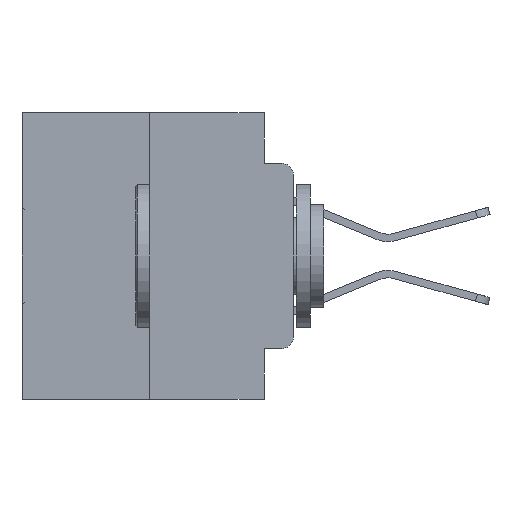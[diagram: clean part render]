
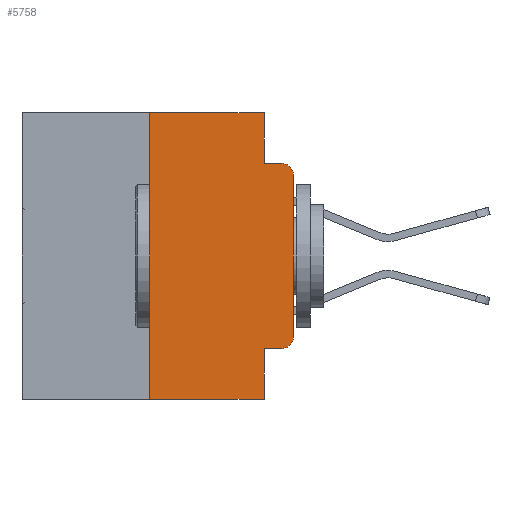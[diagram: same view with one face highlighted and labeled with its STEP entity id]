
A CAD part, left-side view. The second image highlights one B-rep face of the part: STEP entity #5758.
In plain terms, the highlighted planar face has unit normal (-1, 0, 0).
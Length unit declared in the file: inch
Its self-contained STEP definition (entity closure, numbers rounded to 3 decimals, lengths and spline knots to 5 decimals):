
#110 = ORIENTED_EDGE ( 'NONE', *, *, #951, .T. ) ;
#783 = VERTEX_POINT ( 'NONE', #11656 ) ;
#951 = EDGE_CURVE ( 'NONE', #11576, #783, #6256, .T. ) ;
#1330 = CARTESIAN_POINT ( 'NONE',  ( 0., 0., -0.1085 ) ) ;
#1408 = CARTESIAN_POINT ( 'NONE',  ( 0., 0.051, -0.4115 ) ) ;
#1861 = DIRECTION ( 'NONE',  ( 0., -1., 0. ) ) ;
#2162 = LINE ( 'NONE', #21679, #14108 ) ;
#2329 = ORIENTED_EDGE ( 'NONE', *, *, #25885, .T. ) ;
#2537 = ORIENTED_EDGE ( 'NONE', *, *, #22961, .T. ) ;
#3094 = VECTOR ( 'NONE', #11346, 39.37008 ) ;
#3919 = CARTESIAN_POINT ( 'NONE',  ( 0., 0.051, 0. ) ) ;
#4466 = ORIENTED_EDGE ( 'NONE', *, *, #26019, .F. ) ;
#4568 = VERTEX_POINT ( 'NONE', #19889 ) ;
#4590 = CARTESIAN_POINT ( 'NONE',  ( 0., 0.051, -0.0885 ) ) ;
#4598 = VECTOR ( 'NONE', #23918, 39.37008 ) ;
#4749 = LINE ( 'NONE', #4590, #29513 ) ;
#4947 = VECTOR ( 'NONE', #23850, 39.37008 ) ;
#5652 = CARTESIAN_POINT ( 'NONE',  ( 0., 0.473, 0. ) ) ;
#5730 = VERTEX_POINT ( 'NONE', #3919 ) ;
#5758 = ADVANCED_FACE ( 'NONE', ( #13827 ), #16382, .F. ) ;
#6256 = CIRCLE ( 'NONE', #24611, 0.02 ) ;
#6476 = VERTEX_POINT ( 'NONE', #13282 ) ;
#6518 = CARTESIAN_POINT ( 'NONE',  ( 0., 0.051, 0. ) ) ;
#6562 = ORIENTED_EDGE ( 'NONE', *, *, #10636, .T. ) ;
#7818 = DIRECTION ( 'NONE',  ( -1., 0., 0. ) ) ;
#8045 = AXIS2_PLACEMENT_3D ( 'NONE', #23217, #16023, #23375 ) ;
#8995 = VECTOR ( 'NONE', #14072, 39.37008 ) ;
#10472 = VERTEX_POINT ( 'NONE', #24785 ) ;
#10501 = VERTEX_POINT ( 'NONE', #22683 ) ;
#10636 = EDGE_CURVE ( 'NONE', #4568, #10501, #28134, .T. ) ;
#10892 = EDGE_LOOP ( 'NONE', ( #24279, #110, #16818, #15196, #11909, #19947, #2537, #4466, #6562, #2329 ) ) ;
#11265 = EDGE_CURVE ( 'NONE', #5730, #23530, #21369, .T. ) ;
#11346 = DIRECTION ( 'NONE',  ( 0., -1., 0. ) ) ;
#11576 = VERTEX_POINT ( 'NONE', #1330 ) ;
#11656 = CARTESIAN_POINT ( 'NONE',  ( 0., 0.02, -0.0885 ) ) ;
#11909 = ORIENTED_EDGE ( 'NONE', *, *, #29286, .F. ) ;
#13282 = CARTESIAN_POINT ( 'NONE',  ( 0., 0.051, -0.5 ) ) ;
#13827 = FACE_OUTER_BOUND ( 'NONE', #10892, .T. ) ;
#14072 = DIRECTION ( 'NONE',  ( 0., -1., 0. ) ) ;
#14108 = VECTOR ( 'NONE', #24236, 39.37008 ) ;
#14802 = VERTEX_POINT ( 'NONE', #14879 ) ;
#14879 = CARTESIAN_POINT ( 'NONE',  ( 0., 0., -0.3915 ) ) ;
#15196 = ORIENTED_EDGE ( 'NONE', *, *, #11265, .F. ) ;
#15603 = CARTESIAN_POINT ( 'NONE',  ( 0., 0.051, -0.0885 ) ) ;
#16003 = CARTESIAN_POINT ( 'NONE',  ( 0., 0.473, -0.5 ) ) ;
#16023 = DIRECTION ( 'NONE',  ( -1., 0., 0. ) ) ;
#16382 = PLANE ( 'NONE',  #30976 ) ;
#16492 = LINE ( 'NONE', #31544, #4947 ) ;
#16818 = ORIENTED_EDGE ( 'NONE', *, *, #20295, .F. ) ;
#17702 = DIRECTION ( 'NONE',  ( 0., 0., -1. ) ) ;
#17843 = LINE ( 'NONE', #22940, #27909 ) ;
#19107 = DIRECTION ( 'NONE',  ( 0., 0., -1. ) ) ;
#19286 = EDGE_CURVE ( 'NONE', #26564, #10472, #17843, .T. ) ;
#19883 = LINE ( 'NONE', #5652, #29651 ) ;
#19889 = CARTESIAN_POINT ( 'NONE',  ( 0., 0.051, -0.4115 ) ) ;
#19947 = ORIENTED_EDGE ( 'NONE', *, *, #19286, .F. ) ;
#20295 = EDGE_CURVE ( 'NONE', #23530, #783, #4749, .T. ) ;
#21027 = DIRECTION ( 'NONE',  ( 1., 0., 0. ) ) ;
#21369 = LINE ( 'NONE', #6518, #4598 ) ;
#21679 = CARTESIAN_POINT ( 'NONE',  ( 0., 0., 0. ) ) ;
#22683 = CARTESIAN_POINT ( 'NONE',  ( 0., 0.02, -0.4115 ) ) ;
#22940 = CARTESIAN_POINT ( 'NONE',  ( 0., 0.25, 0. ) ) ;
#22961 = EDGE_CURVE ( 'NONE', #26564, #6476, #28492, .T. ) ;
#23217 = CARTESIAN_POINT ( 'NONE',  ( 0., 0.02, -0.3915 ) ) ;
#23375 = DIRECTION ( 'NONE',  ( 0., 0., -1. ) ) ;
#23530 = VERTEX_POINT ( 'NONE', #15603 ) ;
#23582 = EDGE_CURVE ( 'NONE', #14802, #11576, #2162, .T. ) ;
#23850 = DIRECTION ( 'NONE',  ( 0., 0., -1. ) ) ;
#23918 = DIRECTION ( 'NONE',  ( 0., 0., -1. ) ) ;
#24236 = DIRECTION ( 'NONE',  ( 0., 0., 1. ) ) ;
#24279 = ORIENTED_EDGE ( 'NONE', *, *, #23582, .T. ) ;
#24346 = CIRCLE ( 'NONE', #8045, 0.02 ) ;
#24611 = AXIS2_PLACEMENT_3D ( 'NONE', #24755, #7818, #17702 ) ;
#24755 = CARTESIAN_POINT ( 'NONE',  ( 0., 0.02, -0.1085 ) ) ;
#24785 = CARTESIAN_POINT ( 'NONE',  ( 0., 0.25, 0. ) ) ;
#24838 = DIRECTION ( 'NONE',  ( 0., -1., 0. ) ) ;
#24920 = CARTESIAN_POINT ( 'NONE',  ( 0., 0.25, -0.5 ) ) ;
#25885 = EDGE_CURVE ( 'NONE', #10501, #14802, #24346, .T. ) ;
#26019 = EDGE_CURVE ( 'NONE', #4568, #6476, #16492, .T. ) ;
#26147 = CARTESIAN_POINT ( 'NONE',  ( 0., 0.473, 0. ) ) ;
#26564 = VERTEX_POINT ( 'NONE', #24920 ) ;
#27606 = DIRECTION ( 'NONE',  ( 0., 0., 1. ) ) ;
#27909 = VECTOR ( 'NONE', #27606, 39.37008 ) ;
#28134 = LINE ( 'NONE', #1408, #3094 ) ;
#28492 = LINE ( 'NONE', #16003, #8995 ) ;
#29286 = EDGE_CURVE ( 'NONE', #10472, #5730, #19883, .T. ) ;
#29513 = VECTOR ( 'NONE', #1861, 39.37008 ) ;
#29651 = VECTOR ( 'NONE', #24838, 39.37008 ) ;
#30976 = AXIS2_PLACEMENT_3D ( 'NONE', #26147, #21027, #19107 ) ;
#31544 = CARTESIAN_POINT ( 'NONE',  ( 0., 0.051, 0. ) ) ;
